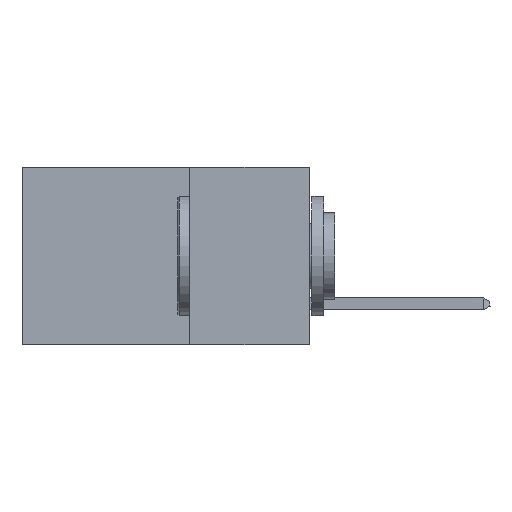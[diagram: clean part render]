
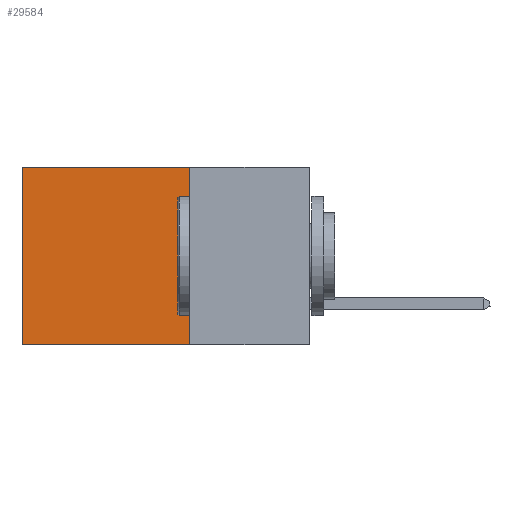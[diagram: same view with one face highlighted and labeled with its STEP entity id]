
A CAD part, left-side view. The second image highlights one B-rep face of the part: STEP entity #29584.
In plain terms, the highlighted planar face has unit normal (-1, 0, 0).
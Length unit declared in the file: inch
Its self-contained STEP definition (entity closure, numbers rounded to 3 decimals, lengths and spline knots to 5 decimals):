
#1316 = EDGE_CURVE ( 'NONE', #16107, #21655, #35824, .T. ) ;
#1424 = CARTESIAN_POINT ( 'NONE',  ( 0.2875, 0.25, 0. ) ) ;
#2428 = LINE ( 'NONE', #20030, #40571 ) ;
#4862 = ORIENTED_EDGE ( 'NONE', *, *, #13505, .F. ) ;
#4949 = VECTOR ( 'NONE', #7797, 39.37008 ) ;
#7398 = AXIS2_PLACEMENT_3D ( 'NONE', #1424, #36126, #8404 ) ;
#7797 = DIRECTION ( 'NONE',  ( 0., 0., -1. ) ) ;
#8404 = DIRECTION ( 'NONE',  ( 0., 0., -1. ) ) ;
#8775 = EDGE_CURVE ( 'NONE', #30986, #21655, #25925, .T. ) ;
#10853 = DIRECTION ( 'NONE',  ( 0., 1., 0. ) ) ;
#12751 = ORIENTED_EDGE ( 'NONE', *, *, #17943, .T. ) ;
#12862 = LINE ( 'NONE', #21484, #23949 ) ;
#13505 = EDGE_CURVE ( 'NONE', #18342, #16107, #2428, .T. ) ;
#15205 = PLANE ( 'NONE',  #7398 ) ;
#16107 = VERTEX_POINT ( 'NONE', #40367 ) ;
#16970 = CARTESIAN_POINT ( 'NONE',  ( 0.2875, 0.6, 0. ) ) ;
#17943 = EDGE_CURVE ( 'NONE', #18342, #30986, #12862, .T. ) ;
#17971 = CARTESIAN_POINT ( 'NONE',  ( 0.2875, 0.25, -0.37 ) ) ;
#18342 = VERTEX_POINT ( 'NONE', #21275 ) ;
#20030 = CARTESIAN_POINT ( 'NONE',  ( 0.2875, 0.25, 0. ) ) ;
#20928 = DIRECTION ( 'NONE',  ( 0., 0., -1. ) ) ;
#21275 = CARTESIAN_POINT ( 'NONE',  ( 0.2875, 0.25, 0. ) ) ;
#21484 = CARTESIAN_POINT ( 'NONE',  ( 0.2875, 0.25, 0. ) ) ;
#21655 = VERTEX_POINT ( 'NONE', #44528 ) ;
#23949 = VECTOR ( 'NONE', #43161, 39.37008 ) ;
#25925 = LINE ( 'NONE', #39001, #4949 ) ;
#29584 = ADVANCED_FACE ( 'NONE', ( #34157 ), #15205, .F. ) ;
#30986 = VERTEX_POINT ( 'NONE', #16970 ) ;
#31137 = ORIENTED_EDGE ( 'NONE', *, *, #8775, .T. ) ;
#34157 = FACE_OUTER_BOUND ( 'NONE', #45695, .T. ) ;
#35266 = VECTOR ( 'NONE', #10853, 39.37008 ) ;
#35824 = LINE ( 'NONE', #17971, #35266 ) ;
#36126 = DIRECTION ( 'NONE',  ( 1., 0., 0. ) ) ;
#39001 = CARTESIAN_POINT ( 'NONE',  ( 0.2875, 0.6, 0. ) ) ;
#40367 = CARTESIAN_POINT ( 'NONE',  ( 0.2875, 0.25, -0.37 ) ) ;
#40571 = VECTOR ( 'NONE', #20928, 39.37008 ) ;
#42286 = ORIENTED_EDGE ( 'NONE', *, *, #1316, .F. ) ;
#43161 = DIRECTION ( 'NONE',  ( 0., 1., 0. ) ) ;
#44528 = CARTESIAN_POINT ( 'NONE',  ( 0.2875, 0.6, -0.37 ) ) ;
#45695 = EDGE_LOOP ( 'NONE', ( #31137, #42286, #4862, #12751 ) ) ;
